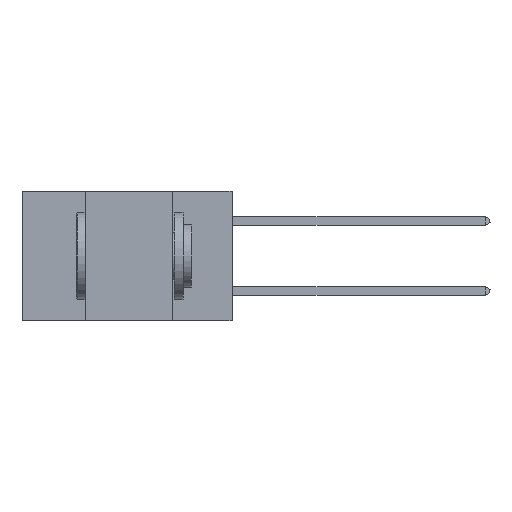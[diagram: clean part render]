
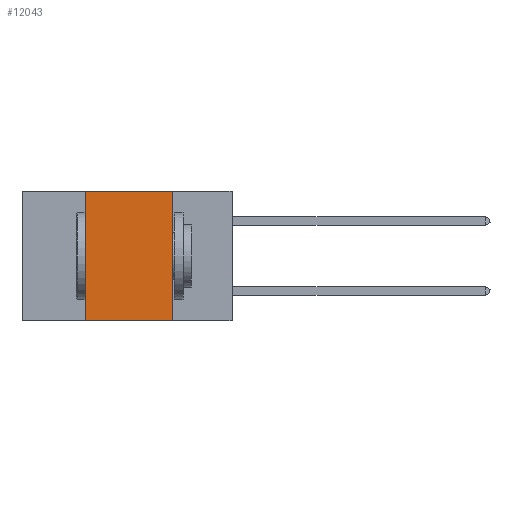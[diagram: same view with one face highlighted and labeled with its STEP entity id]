
A CAD part, left-side view. The second image highlights one B-rep face of the part: STEP entity #12043.
In plain terms, the highlighted planar face has unit normal (-1, 0, 0).
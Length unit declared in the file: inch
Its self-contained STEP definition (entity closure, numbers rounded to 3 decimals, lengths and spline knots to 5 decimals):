
#148 = CARTESIAN_POINT ( 'NONE',  ( 0., 0.17, -0.37 ) ) ;
#385 = LINE ( 'NONE', #7797, #18179 ) ;
#1121 = DIRECTION ( 'NONE',  ( 0., 0., 1. ) ) ;
#3660 = CARTESIAN_POINT ( 'NONE',  ( 0., 0.6, 0. ) ) ;
#3996 = CARTESIAN_POINT ( 'NONE',  ( 0., 0.6, -0.37 ) ) ;
#4706 = VERTEX_POINT ( 'NONE', #148 ) ;
#4793 = VECTOR ( 'NONE', #1121, 39.37008 ) ;
#5561 = PLANE ( 'NONE',  #9079 ) ;
#5806 = DIRECTION ( 'NONE',  ( 0., -1., 0. ) ) ;
#6173 = ORIENTED_EDGE ( 'NONE', *, *, #12020, .F. ) ;
#6528 = EDGE_CURVE ( 'NONE', #12223, #17439, #22075, .T. ) ;
#7388 = DIRECTION ( 'NONE',  ( 1., 0., 0. ) ) ;
#7797 = CARTESIAN_POINT ( 'NONE',  ( 0., 0.17, 0. ) ) ;
#8312 = FACE_OUTER_BOUND ( 'NONE', #13120, .T. ) ;
#8521 = CARTESIAN_POINT ( 'NONE',  ( 0., 0.17, 0. ) ) ;
#9079 = AXIS2_PLACEMENT_3D ( 'NONE', #17404, #7388, #19020 ) ;
#9440 = EDGE_CURVE ( 'NONE', #20817, #4706, #385, .T. ) ;
#10821 = ORIENTED_EDGE ( 'NONE', *, *, #6528, .F. ) ;
#12020 = EDGE_CURVE ( 'NONE', #17439, #20817, #21973, .T. ) ;
#12043 = ADVANCED_FACE ( 'NONE', ( #8312 ), #5561, .F. ) ;
#12223 = VERTEX_POINT ( 'NONE', #17835 ) ;
#12837 = VECTOR ( 'NONE', #20412, 39.37008 ) ;
#13120 = EDGE_LOOP ( 'NONE', ( #19026, #6173, #10821, #19536 ) ) ;
#13909 = CARTESIAN_POINT ( 'NONE',  ( 0., 0.42, 0. ) ) ;
#14635 = LINE ( 'NONE', #3996, #18452 ) ;
#16201 = DIRECTION ( 'NONE',  ( 0., 0., -1. ) ) ;
#17404 = CARTESIAN_POINT ( 'NONE',  ( 0., 0.6, 0. ) ) ;
#17439 = VERTEX_POINT ( 'NONE', #13909 ) ;
#17835 = CARTESIAN_POINT ( 'NONE',  ( 0., 0.42, -0.37 ) ) ;
#18179 = VECTOR ( 'NONE', #16201, 39.37008 ) ;
#18452 = VECTOR ( 'NONE', #5806, 39.37008 ) ;
#19020 = DIRECTION ( 'NONE',  ( 0., 0., -1. ) ) ;
#19026 = ORIENTED_EDGE ( 'NONE', *, *, #9440, .F. ) ;
#19446 = EDGE_CURVE ( 'NONE', #12223, #4706, #14635, .T. ) ;
#19536 = ORIENTED_EDGE ( 'NONE', *, *, #19446, .T. ) ;
#20412 = DIRECTION ( 'NONE',  ( 0., -1., 0. ) ) ;
#20817 = VERTEX_POINT ( 'NONE', #8521 ) ;
#21540 = CARTESIAN_POINT ( 'NONE',  ( 0., 0.42, 0. ) ) ;
#21973 = LINE ( 'NONE', #3660, #12837 ) ;
#22075 = LINE ( 'NONE', #21540, #4793 ) ;
